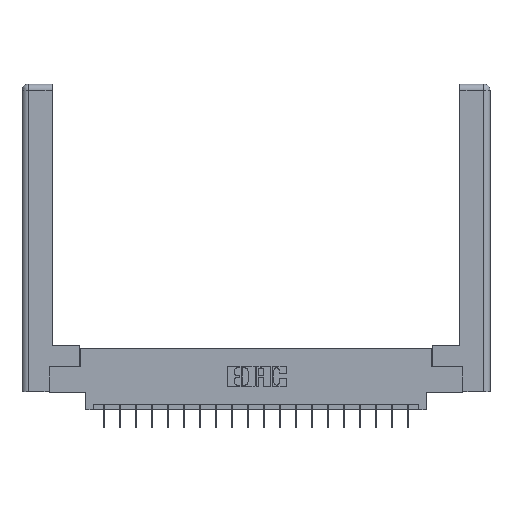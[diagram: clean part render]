
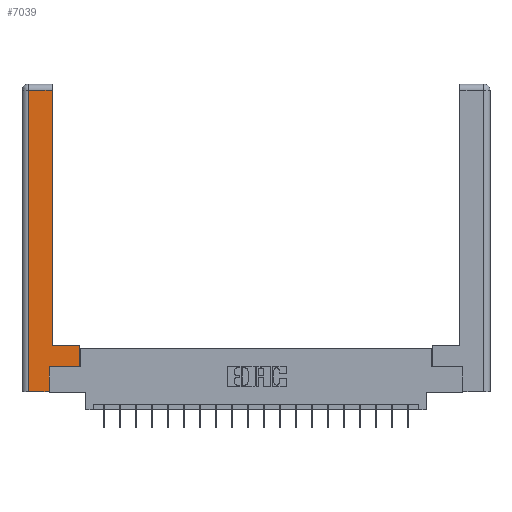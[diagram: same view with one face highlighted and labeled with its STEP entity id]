
A CAD part, top view. The second image highlights one B-rep face of the part: STEP entity #7039.
In plain terms, the highlighted planar face has unit normal (0, 0, 1).
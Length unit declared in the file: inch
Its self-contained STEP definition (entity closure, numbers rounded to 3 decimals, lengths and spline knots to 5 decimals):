
#16 = ORIENTED_EDGE ( 'NONE', *, *, #8291, .T. ) ;
#166 = AXIS2_PLACEMENT_3D ( 'NONE', #14003, #12495, #5808 ) ;
#253 = ORIENTED_EDGE ( 'NONE', *, *, #10895, .T. ) ;
#328 = LINE ( 'NONE', #1849, #20293 ) ;
#926 = CARTESIAN_POINT ( 'NONE',  ( 0.265, 0.245, 0. ) ) ;
#1695 = DIRECTION ( 'NONE',  ( -1., 0., 0. ) ) ;
#1849 = CARTESIAN_POINT ( 'NONE',  ( 0.295, 0.45, 0. ) ) ;
#2135 = CARTESIAN_POINT ( 'NONE',  ( 0.265, 0., 0. ) ) ;
#2407 = CARTESIAN_POINT ( 'NONE',  ( 0.0615, 2.94, 0. ) ) ;
#2453 = LINE ( 'NONE', #5128, #12701 ) ;
#2709 = DIRECTION ( 'NONE',  ( 0., 1., 0. ) ) ;
#2755 = CARTESIAN_POINT ( 'NONE',  ( 0.565, 0.45, 0. ) ) ;
#2791 = VERTEX_POINT ( 'NONE', #7429 ) ;
#3859 = LINE ( 'NONE', #20685, #12077 ) ;
#3993 = ORIENTED_EDGE ( 'NONE', *, *, #8804, .T. ) ;
#4290 = VERTEX_POINT ( 'NONE', #5252 ) ;
#4522 = CARTESIAN_POINT ( 'NONE',  ( 0.565, 0.245, 0. ) ) ;
#5009 = LINE ( 'NONE', #12118, #6544 ) ;
#5028 = VERTEX_POINT ( 'NONE', #2755 ) ;
#5083 = VECTOR ( 'NONE', #2709, 39.37008 ) ;
#5128 = CARTESIAN_POINT ( 'NONE',  ( 0.565, 0.45, 0. ) ) ;
#5252 = CARTESIAN_POINT ( 'NONE',  ( 0.265, 0.245, 0. ) ) ;
#5577 = DIRECTION ( 'NONE',  ( -1., 0., 0. ) ) ;
#5808 = DIRECTION ( 'NONE',  ( -1., 0., 0. ) ) ;
#6544 = VECTOR ( 'NONE', #5577, 39.37008 ) ;
#6751 = EDGE_CURVE ( 'NONE', #5028, #14080, #328, .T. ) ;
#7039 = ADVANCED_FACE ( 'NONE', ( #13102 ), #19023, .F. ) ;
#7121 = DIRECTION ( 'NONE',  ( 1., 0., 0. ) ) ;
#7429 = CARTESIAN_POINT ( 'NONE',  ( 0.265, 0., 0. ) ) ;
#7633 = ORIENTED_EDGE ( 'NONE', *, *, #6751, .T. ) ;
#8051 = CARTESIAN_POINT ( 'NONE',  ( 0.0615, 0., 0. ) ) ;
#8291 = EDGE_CURVE ( 'NONE', #2791, #4290, #19951, .T. ) ;
#8473 = EDGE_CURVE ( 'NONE', #13067, #13862, #9968, .T. ) ;
#8532 = ORIENTED_EDGE ( 'NONE', *, *, #14300, .T. ) ;
#8804 = EDGE_CURVE ( 'NONE', #13862, #2791, #18393, .T. ) ;
#9545 = DIRECTION ( 'NONE',  ( 1., 0., 0. ) ) ;
#9968 = LINE ( 'NONE', #8051, #17136 ) ;
#10895 = EDGE_CURVE ( 'NONE', #19043, #13067, #5009, .T. ) ;
#11243 = VECTOR ( 'NONE', #7121, 39.37008 ) ;
#11508 = CARTESIAN_POINT ( 'NONE',  ( 0.295, 2.94, 0. ) ) ;
#11643 = ORIENTED_EDGE ( 'NONE', *, *, #13390, .T. ) ;
#11812 = CARTESIAN_POINT ( 'NONE',  ( 0.565, 0.245, 0. ) ) ;
#12001 = ORIENTED_EDGE ( 'NONE', *, *, #8473, .T. ) ;
#12077 = VECTOR ( 'NONE', #15665, 39.37008 ) ;
#12118 = CARTESIAN_POINT ( 'NONE',  ( 0.0615, 2.94, 0. ) ) ;
#12495 = DIRECTION ( 'NONE',  ( 0., 0., -1. ) ) ;
#12701 = VECTOR ( 'NONE', #16594, 39.37008 ) ;
#13067 = VERTEX_POINT ( 'NONE', #2407 ) ;
#13102 = FACE_OUTER_BOUND ( 'NONE', #21188, .T. ) ;
#13390 = EDGE_CURVE ( 'NONE', #4290, #14344, #20176, .T. ) ;
#13862 = VERTEX_POINT ( 'NONE', #15465 ) ;
#14003 = CARTESIAN_POINT ( 'NONE',  ( 0., 0., 0. ) ) ;
#14080 = VERTEX_POINT ( 'NONE', #16313 ) ;
#14300 = EDGE_CURVE ( 'NONE', #14344, #5028, #2453, .T. ) ;
#14344 = VERTEX_POINT ( 'NONE', #11812 ) ;
#15465 = CARTESIAN_POINT ( 'NONE',  ( 0.0615, 0., 0. ) ) ;
#15665 = DIRECTION ( 'NONE',  ( 0., 1., 0. ) ) ;
#16084 = DIRECTION ( 'NONE',  ( 0., -1., 0. ) ) ;
#16313 = CARTESIAN_POINT ( 'NONE',  ( 0.295, 0.45, 0. ) ) ;
#16594 = DIRECTION ( 'NONE',  ( 0., 1., 0. ) ) ;
#16844 = VECTOR ( 'NONE', #9545, 39.37008 ) ;
#17136 = VECTOR ( 'NONE', #16084, 39.37008 ) ;
#18393 = LINE ( 'NONE', #2135, #11243 ) ;
#19023 = PLANE ( 'NONE',  #166 ) ;
#19043 = VERTEX_POINT ( 'NONE', #11508 ) ;
#19951 = LINE ( 'NONE', #926, #5083 ) ;
#20043 = EDGE_CURVE ( 'NONE', #14080, #19043, #3859, .T. ) ;
#20176 = LINE ( 'NONE', #4522, #16844 ) ;
#20293 = VECTOR ( 'NONE', #1695, 39.37008 ) ;
#20685 = CARTESIAN_POINT ( 'NONE',  ( 0.295, 3., 0. ) ) ;
#20751 = ORIENTED_EDGE ( 'NONE', *, *, #20043, .T. ) ;
#21188 = EDGE_LOOP ( 'NONE', ( #20751, #253, #12001, #3993, #16, #11643, #8532, #7633 ) ) ;
